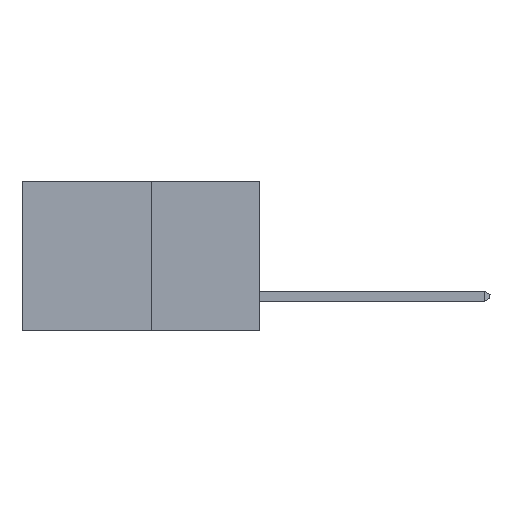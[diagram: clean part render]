
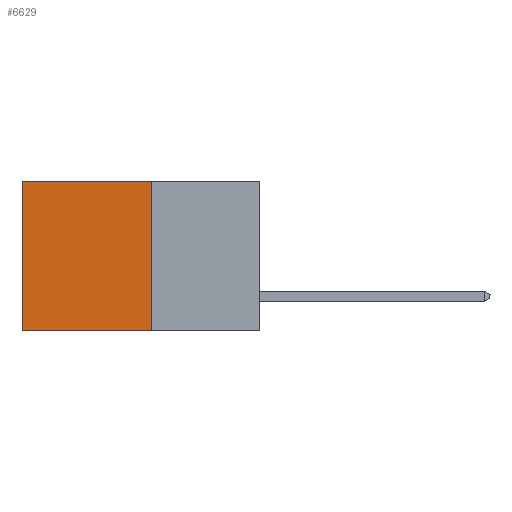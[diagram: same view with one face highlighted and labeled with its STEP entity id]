
A CAD part, left-side view. The second image highlights one B-rep face of the part: STEP entity #6629.
In plain terms, the highlighted planar face has unit normal (-1, 0, 0).
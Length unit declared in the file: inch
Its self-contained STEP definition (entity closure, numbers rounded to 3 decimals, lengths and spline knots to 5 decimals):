
#721 = DIRECTION ( 'NONE',  ( 0., 0., -1. ) ) ;
#1818 = VECTOR ( 'NONE', #721, 39.37008 ) ;
#2488 = LINE ( 'NONE', #17905, #21416 ) ;
#3064 = CARTESIAN_POINT ( 'NONE',  ( 0.277, 0.27, 0. ) ) ;
#4534 = ORIENTED_EDGE ( 'NONE', *, *, #12102, .T. ) ;
#5073 = FACE_OUTER_BOUND ( 'NONE', #19015, .T. ) ;
#6293 = DIRECTION ( 'NONE',  ( 0., 0., -1. ) ) ;
#6629 = ADVANCED_FACE ( 'NONE', ( #5073 ), #8555, .F. ) ;
#7747 = DIRECTION ( 'NONE',  ( 0., 0., -1. ) ) ;
#7766 = VECTOR ( 'NONE', #6293, 39.37008 ) ;
#8104 = CARTESIAN_POINT ( 'NONE',  ( 0.277, 0.59, -0.37 ) ) ;
#8444 = DIRECTION ( 'NONE',  ( 1., 0., 0. ) ) ;
#8447 = CARTESIAN_POINT ( 'NONE',  ( 0.277, 0.27, -0.37 ) ) ;
#8555 = PLANE ( 'NONE',  #18538 ) ;
#9301 = EDGE_CURVE ( 'NONE', #15377, #12453, #2488, .T. ) ;
#9952 = LINE ( 'NONE', #16830, #14300 ) ;
#11637 = VERTEX_POINT ( 'NONE', #12335 ) ;
#12102 = EDGE_CURVE ( 'NONE', #12453, #11637, #22446, .T. ) ;
#12335 = CARTESIAN_POINT ( 'NONE',  ( 0.277, 0.59, -0.37 ) ) ;
#12453 = VERTEX_POINT ( 'NONE', #16463 ) ;
#14291 = ORIENTED_EDGE ( 'NONE', *, *, #16815, .F. ) ;
#14300 = VECTOR ( 'NONE', #18672, 39.37008 ) ;
#15377 = VERTEX_POINT ( 'NONE', #3064 ) ;
#15460 = ORIENTED_EDGE ( 'NONE', *, *, #19668, .F. ) ;
#16054 = VERTEX_POINT ( 'NONE', #18389 ) ;
#16463 = CARTESIAN_POINT ( 'NONE',  ( 0.277, 0.59, 0. ) ) ;
#16505 = LINE ( 'NONE', #22695, #1818 ) ;
#16661 = ORIENTED_EDGE ( 'NONE', *, *, #9301, .T. ) ;
#16815 = EDGE_CURVE ( 'NONE', #16054, #11637, #9952, .T. ) ;
#16830 = CARTESIAN_POINT ( 'NONE',  ( 0.277, 0.27, -0.37 ) ) ;
#17905 = CARTESIAN_POINT ( 'NONE',  ( 0.277, 0.27, 0. ) ) ;
#18389 = CARTESIAN_POINT ( 'NONE',  ( 0.277, 0.27, -0.37 ) ) ;
#18538 = AXIS2_PLACEMENT_3D ( 'NONE', #8447, #8444, #7747 ) ;
#18672 = DIRECTION ( 'NONE',  ( 0., 1., 0. ) ) ;
#19015 = EDGE_LOOP ( 'NONE', ( #4534, #14291, #15460, #16661 ) ) ;
#19668 = EDGE_CURVE ( 'NONE', #15377, #16054, #16505, .T. ) ;
#19693 = DIRECTION ( 'NONE',  ( 0., 1., 0. ) ) ;
#21416 = VECTOR ( 'NONE', #19693, 39.37008 ) ;
#22446 = LINE ( 'NONE', #8104, #7766 ) ;
#22695 = CARTESIAN_POINT ( 'NONE',  ( 0.277, 0.27, -0.37 ) ) ;
